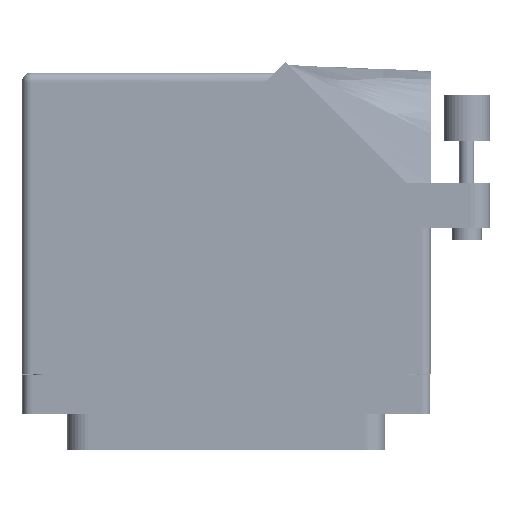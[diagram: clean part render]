
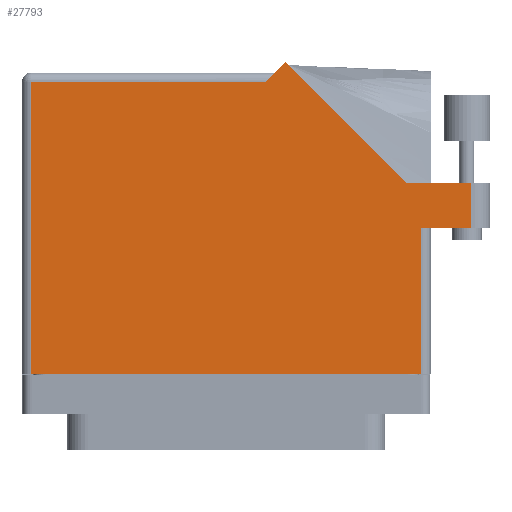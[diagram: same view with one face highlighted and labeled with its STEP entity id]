
A CAD part, front view. The second image highlights one B-rep face of the part: STEP entity #27793.
In plain terms, the highlighted face is planar.
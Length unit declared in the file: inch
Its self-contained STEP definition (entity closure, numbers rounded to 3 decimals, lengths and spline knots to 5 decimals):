
#296 = LINE ( 'NONE', #25182, #73649 ) ;
#1575 = CARTESIAN_POINT ( 'NONE',  ( 1.3155, 0.88, 0.765 ) ) ;
#3804 = CARTESIAN_POINT ( 'NONE',  ( 0.3275, 1.93, 0.765 ) ) ;
#3923 = EDGE_CURVE ( 'NONE', #59827, #21025, #76699, .T. ) ;
#4159 = VECTOR ( 'NONE', #34318, 39.37008 ) ;
#6007 = CARTESIAN_POINT ( 'NONE',  ( -1.3155, 1.868, 0.765 ) ) ;
#7388 = CARTESIAN_POINT ( 'NONE',  ( -1.3155, -0.1, 0.765 ) ) ;
#8185 = ORIENTED_EDGE ( 'NONE', *, *, #83601, .T. ) ;
#8522 = CARTESIAN_POINT ( 'NONE',  ( 1.7775, 1.187, 0.765 ) ) ;
#9507 = VERTEX_POINT ( 'NONE', #19746 ) ;
#9620 = ORIENTED_EDGE ( 'NONE', *, *, #72934, .T. ) ;
#9806 = AXIS2_PLACEMENT_3D ( 'NONE', #82033, #12444, #60716 ) ;
#9909 = ORIENTED_EDGE ( 'NONE', *, *, #3923, .T. ) ;
#10118 = EDGE_CURVE ( 'NONE', #21025, #39128, #30357, .T. ) ;
#10760 = DIRECTION ( 'NONE',  ( -0.707, -0.707, 0. ) ) ;
#11678 = EDGE_CURVE ( 'NONE', #33931, #23904, #59217, .T. ) ;
#12146 = DIRECTION ( 'NONE',  ( -1., 0., 0. ) ) ;
#12444 = DIRECTION ( 'NONE',  ( 0., 0., -1. ) ) ;
#16424 = FACE_OUTER_BOUND ( 'NONE', #41350, .T. ) ;
#18208 = CARTESIAN_POINT ( 'NONE',  ( 1.6525, 1.187, 0.765 ) ) ;
#18762 = CARTESIAN_POINT ( 'NONE',  ( -1.3775, 1.868, 0.765 ) ) ;
#18937 = VERTEX_POINT ( 'NONE', #70915 ) ;
#19554 = CARTESIAN_POINT ( 'NONE',  ( 0.39821, 2.00071, 0.765 ) ) ;
#19746 = CARTESIAN_POINT ( 'NONE',  ( 1.6525, 0.88, 0.765 ) ) ;
#21025 = VERTEX_POINT ( 'NONE', #76355 ) ;
#22341 = LINE ( 'NONE', #74155, #54730 ) ;
#22856 = EDGE_CURVE ( 'NONE', #9507, #18937, #30261, .T. ) ;
#23904 = VERTEX_POINT ( 'NONE', #50688 ) ;
#25182 = CARTESIAN_POINT ( 'NONE',  ( 1.21192, 1.187, 0.765 ) ) ;
#26240 = VERTEX_POINT ( 'NONE', #55519 ) ;
#27793 = ADVANCED_FACE ( 'NONE', ( #16424 ), #61583, .F. ) ;
#30261 = LINE ( 'NONE', #18208, #52965 ) ;
#30357 = LINE ( 'NONE', #18762, #63806 ) ;
#32599 = CARTESIAN_POINT ( 'NONE',  ( -1.3155, -0.1, 0.765 ) ) ;
#33061 = DIRECTION ( 'NONE',  ( -0.707, 0.707, 0. ) ) ;
#33931 = VERTEX_POINT ( 'NONE', #7388 ) ;
#34318 = DIRECTION ( 'NONE',  ( 1., 0., 0. ) ) ;
#35341 = ORIENTED_EDGE ( 'NONE', *, *, #11678, .T. ) ;
#37628 = ORIENTED_EDGE ( 'NONE', *, *, #52379, .T. ) ;
#39128 = VERTEX_POINT ( 'NONE', #6007 ) ;
#39207 = DIRECTION ( 'NONE',  ( 0., -1., 0. ) ) ;
#41350 = EDGE_LOOP ( 'NONE', ( #79565, #68417, #37628, #9620, #9909, #84689, #8185, #35341, #46988 ) ) ;
#43779 = DIRECTION ( 'NONE',  ( -1., 0., 0. ) ) ;
#45157 = VERTEX_POINT ( 'NONE', #83871 ) ;
#46599 = DIRECTION ( 'NONE',  ( 0., 1., 0. ) ) ;
#46988 = ORIENTED_EDGE ( 'NONE', *, *, #61444, .T. ) ;
#47610 = CARTESIAN_POINT ( 'NONE',  ( -1.3775, -0.1, 0.765 ) ) ;
#50688 = CARTESIAN_POINT ( 'NONE',  ( 1.3155, -0.1, 0.765 ) ) ;
#52379 = EDGE_CURVE ( 'NONE', #18937, #26240, #53794, .T. ) ;
#52737 = EDGE_CURVE ( 'NONE', #45157, #9507, #22341, .T. ) ;
#52965 = VECTOR ( 'NONE', #46599, 39.37008 ) ;
#53794 = LINE ( 'NONE', #8522, #89354 ) ;
#54730 = VECTOR ( 'NONE', #75666, 39.37008 ) ;
#55519 = CARTESIAN_POINT ( 'NONE',  ( 1.21192, 1.187, 0.765 ) ) ;
#57374 = DIRECTION ( 'NONE',  ( 0., 1., 0. ) ) ;
#59217 = LINE ( 'NONE', #47610, #4159 ) ;
#59553 = VECTOR ( 'NONE', #10760, 39.37008 ) ;
#59827 = VERTEX_POINT ( 'NONE', #19554 ) ;
#60716 = DIRECTION ( 'NONE',  ( -1., 0., 0. ) ) ;
#60718 = VECTOR ( 'NONE', #39207, 39.37008 ) ;
#61251 = VECTOR ( 'NONE', #57374, 39.37008 ) ;
#61444 = EDGE_CURVE ( 'NONE', #23904, #45157, #65527, .T. ) ;
#61583 = PLANE ( 'NONE',  #9806 ) ;
#63806 = VECTOR ( 'NONE', #12146, 39.37008 ) ;
#65527 = LINE ( 'NONE', #1575, #61251 ) ;
#68417 = ORIENTED_EDGE ( 'NONE', *, *, #22856, .T. ) ;
#70915 = CARTESIAN_POINT ( 'NONE',  ( 1.6525, 1.187, 0.765 ) ) ;
#72934 = EDGE_CURVE ( 'NONE', #26240, #59827, #296, .T. ) ;
#73649 = VECTOR ( 'NONE', #33061, 39.37008 ) ;
#74155 = CARTESIAN_POINT ( 'NONE',  ( 1.3775, 0.88, 0.765 ) ) ;
#75666 = DIRECTION ( 'NONE',  ( 1., 0., 0. ) ) ;
#76355 = CARTESIAN_POINT ( 'NONE',  ( 0.2655, 1.868, 0.765 ) ) ;
#76699 = LINE ( 'NONE', #3804, #59553 ) ;
#79565 = ORIENTED_EDGE ( 'NONE', *, *, #52737, .T. ) ;
#82033 = CARTESIAN_POINT ( 'NONE',  ( -1.3775, 1.93, 0.765 ) ) ;
#83399 = LINE ( 'NONE', #32599, #60718 ) ;
#83601 = EDGE_CURVE ( 'NONE', #39128, #33931, #83399, .T. ) ;
#83871 = CARTESIAN_POINT ( 'NONE',  ( 1.3155, 0.88, 0.765 ) ) ;
#84689 = ORIENTED_EDGE ( 'NONE', *, *, #10118, .T. ) ;
#89354 = VECTOR ( 'NONE', #43779, 39.37008 ) ;
